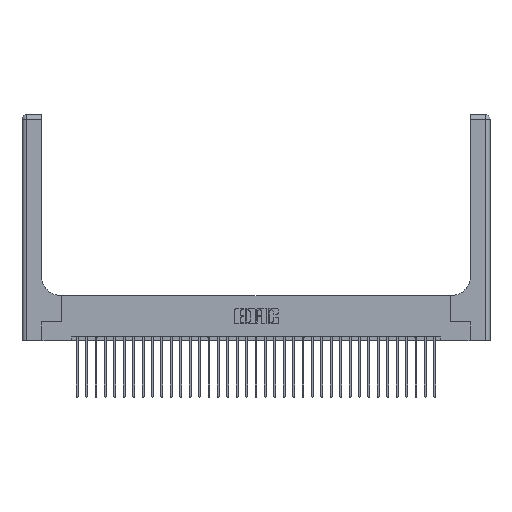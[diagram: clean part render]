
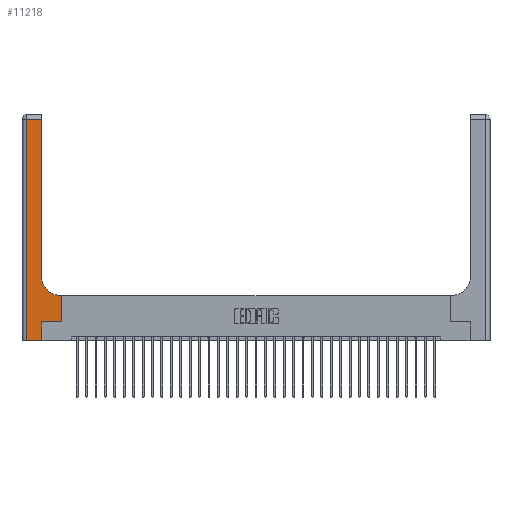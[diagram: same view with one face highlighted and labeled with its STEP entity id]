
A CAD part, top view. The second image highlights one B-rep face of the part: STEP entity #11218.
In plain terms, the highlighted planar face has unit normal (0, 0, 1).
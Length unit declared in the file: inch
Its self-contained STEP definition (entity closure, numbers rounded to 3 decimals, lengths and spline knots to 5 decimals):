
#388 = VERTEX_POINT ( 'NONE', #1727 ) ;
#537 = ORIENTED_EDGE ( 'NONE', *, *, #19831, .T. ) ;
#701 = EDGE_CURVE ( 'NONE', #29399, #388, #25674, .T. ) ;
#887 = LINE ( 'NONE', #10791, #24042 ) ;
#904 = DIRECTION ( 'NONE',  ( -1., 0., 0. ) ) ;
#1218 = CARTESIAN_POINT ( 'NONE',  ( 0.51, 0.85, 0.37 ) ) ;
#1727 = CARTESIAN_POINT ( 'NONE',  ( 0.26, 0.85, 0.37 ) ) ;
#1916 = VERTEX_POINT ( 'NONE', #4291 ) ;
#3362 = ORIENTED_EDGE ( 'NONE', *, *, #6519, .T. ) ;
#3994 = VECTOR ( 'NONE', #30535, 39.37008 ) ;
#4291 = CARTESIAN_POINT ( 'NONE',  ( 0.06, 0., 0.37 ) ) ;
#4874 = LINE ( 'NONE', #22112, #8953 ) ;
#5034 = CARTESIAN_POINT ( 'NONE',  ( 0.06, 3., 0.37 ) ) ;
#5114 = ORIENTED_EDGE ( 'NONE', *, *, #15929, .T. ) ;
#5989 = VECTOR ( 'NONE', #31431, 39.37008 ) ;
#6114 = VECTOR ( 'NONE', #12628, 39.37008 ) ;
#6275 = LINE ( 'NONE', #30213, #3994 ) ;
#6519 = EDGE_CURVE ( 'NONE', #13248, #29399, #18735, .T. ) ;
#6609 = DIRECTION ( 'NONE',  ( -1., 0., 0. ) ) ;
#7428 = VECTOR ( 'NONE', #26434, 39.37008 ) ;
#8188 = VECTOR ( 'NONE', #6609, 39.37008 ) ;
#8374 = EDGE_LOOP ( 'NONE', ( #26513, #5114, #16943, #10610, #23230, #23491, #537, #3362, #17647 ) ) ;
#8953 = VECTOR ( 'NONE', #14128, 39.37008 ) ;
#9043 = DIRECTION ( 'NONE',  ( 0., 0., -1. ) ) ;
#9233 = VERTEX_POINT ( 'NONE', #30976 ) ;
#9437 = LINE ( 'NONE', #21553, #5989 ) ;
#10610 = ORIENTED_EDGE ( 'NONE', *, *, #21937, .T. ) ;
#10659 = CARTESIAN_POINT ( 'NONE',  ( 0., 2.94, 0.37 ) ) ;
#10791 = CARTESIAN_POINT ( 'NONE',  ( 0.26, 3., 0.37 ) ) ;
#10867 = CARTESIAN_POINT ( 'NONE',  ( 0.265, 0., 0.37 ) ) ;
#11218 = ADVANCED_FACE ( 'NONE', ( #28351 ), #28661, .F. ) ;
#11522 = CARTESIAN_POINT ( 'NONE',  ( 0.51, 0.6, 0.37 ) ) ;
#11557 = CARTESIAN_POINT ( 'NONE',  ( 0.06, 2.94, 0.37 ) ) ;
#12245 = EDGE_CURVE ( 'NONE', #9233, #29436, #15337, .T. ) ;
#12628 = DIRECTION ( 'NONE',  ( 0., 1., 0. ) ) ;
#12683 = EDGE_CURVE ( 'NONE', #388, #24793, #887, .T. ) ;
#13248 = VERTEX_POINT ( 'NONE', #25896 ) ;
#13971 = VECTOR ( 'NONE', #904, 39.37008 ) ;
#14067 = CARTESIAN_POINT ( 'NONE',  ( 0.265, 0.25, 0.37 ) ) ;
#14128 = DIRECTION ( 'NONE',  ( 0., 1., 0. ) ) ;
#14292 = LINE ( 'NONE', #5034, #7428 ) ;
#15337 = LINE ( 'NONE', #10867, #6114 ) ;
#15929 = EDGE_CURVE ( 'NONE', #24793, #24531, #25489, .T. ) ;
#16875 = DIRECTION ( 'NONE',  ( -1., 0., 0. ) ) ;
#16943 = ORIENTED_EDGE ( 'NONE', *, *, #19718, .T. ) ;
#17647 = ORIENTED_EDGE ( 'NONE', *, *, #701, .T. ) ;
#18540 = AXIS2_PLACEMENT_3D ( 'NONE', #1218, #25026, #25332 ) ;
#18735 = LINE ( 'NONE', #20665, #8188 ) ;
#19718 = EDGE_CURVE ( 'NONE', #24531, #1916, #14292, .T. ) ;
#19831 = EDGE_CURVE ( 'NONE', #23621, #13248, #4874, .T. ) ;
#20665 = CARTESIAN_POINT ( 'NONE',  ( 0.26, 0.6, 0.37 ) ) ;
#21553 = CARTESIAN_POINT ( 'NONE',  ( 0., 0., 0.37 ) ) ;
#21937 = EDGE_CURVE ( 'NONE', #1916, #9233, #9437, .T. ) ;
#22112 = CARTESIAN_POINT ( 'NONE',  ( 0.528, 0.25, 0.37 ) ) ;
#22886 = CARTESIAN_POINT ( 'NONE',  ( 0.26, 2.94, 0.37 ) ) ;
#23230 = ORIENTED_EDGE ( 'NONE', *, *, #12245, .T. ) ;
#23491 = ORIENTED_EDGE ( 'NONE', *, *, #27704, .T. ) ;
#23587 = CARTESIAN_POINT ( 'NONE',  ( 0., 3., 0.37 ) ) ;
#23621 = VERTEX_POINT ( 'NONE', #28582 ) ;
#24042 = VECTOR ( 'NONE', #25474, 39.37008 ) ;
#24531 = VERTEX_POINT ( 'NONE', #11557 ) ;
#24793 = VERTEX_POINT ( 'NONE', #22886 ) ;
#25026 = DIRECTION ( 'NONE',  ( 0., 0., -1. ) ) ;
#25332 = DIRECTION ( 'NONE',  ( 1., 0., 0. ) ) ;
#25474 = DIRECTION ( 'NONE',  ( 0., 1., 0. ) ) ;
#25489 = LINE ( 'NONE', #10659, #13971 ) ;
#25674 = CIRCLE ( 'NONE', #18540, 0.25 ) ;
#25896 = CARTESIAN_POINT ( 'NONE',  ( 0.528, 0.6, 0.37 ) ) ;
#26434 = DIRECTION ( 'NONE',  ( 0., -1., 0. ) ) ;
#26513 = ORIENTED_EDGE ( 'NONE', *, *, #12683, .T. ) ;
#27704 = EDGE_CURVE ( 'NONE', #29436, #23621, #6275, .T. ) ;
#28351 = FACE_OUTER_BOUND ( 'NONE', #8374, .T. ) ;
#28582 = CARTESIAN_POINT ( 'NONE',  ( 0.528, 0.25, 0.37 ) ) ;
#28661 = PLANE ( 'NONE',  #31498 ) ;
#29399 = VERTEX_POINT ( 'NONE', #11522 ) ;
#29436 = VERTEX_POINT ( 'NONE', #14067 ) ;
#30213 = CARTESIAN_POINT ( 'NONE',  ( 0.265, 0.25, 0.37 ) ) ;
#30535 = DIRECTION ( 'NONE',  ( 1., 0., 0. ) ) ;
#30976 = CARTESIAN_POINT ( 'NONE',  ( 0.265, 0., 0.37 ) ) ;
#31431 = DIRECTION ( 'NONE',  ( 1., 0., 0. ) ) ;
#31498 = AXIS2_PLACEMENT_3D ( 'NONE', #23587, #9043, #16875 ) ;
